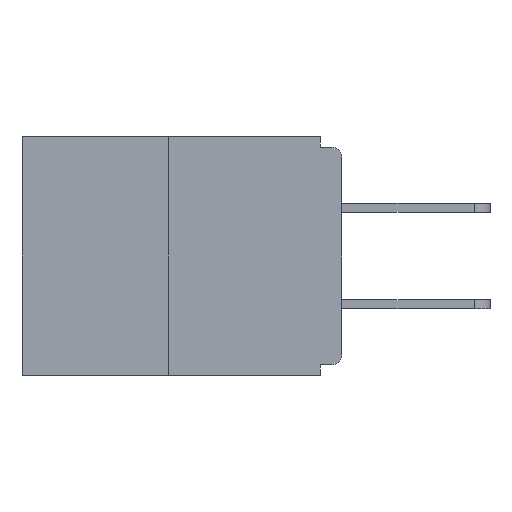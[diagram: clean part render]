
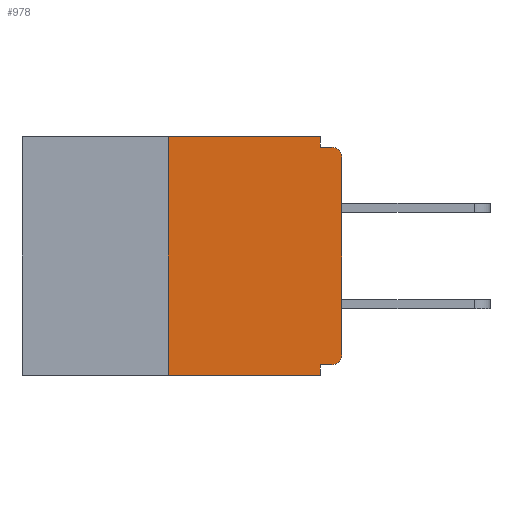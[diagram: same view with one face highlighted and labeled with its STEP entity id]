
A CAD part, left-side view. The second image highlights one B-rep face of the part: STEP entity #978.
In plain terms, the highlighted planar face has unit normal (-1, 0, 0).
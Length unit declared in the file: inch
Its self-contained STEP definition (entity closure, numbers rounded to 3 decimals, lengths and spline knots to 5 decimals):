
#153 = CARTESIAN_POINT ( 'NONE',  ( 0., 0.031, -0.343 ) ) ;
#158 = CARTESIAN_POINT ( 'NONE',  ( 0., 0.25, 0. ) ) ;
#217 = CIRCLE ( 'NONE', #15410, 0.015 ) ;
#261 = DIRECTION ( 'NONE',  ( -1., 0., 0. ) ) ;
#465 = EDGE_CURVE ( 'NONE', #6177, #3303, #217, .T. ) ;
#733 = CARTESIAN_POINT ( 'NONE',  ( 0., 0.46, 0. ) ) ;
#875 = LINE ( 'NONE', #19701, #16586 ) ;
#978 = ADVANCED_FACE ( 'NONE', ( #18193 ), #2371, .F. ) ;
#1172 = LINE ( 'NONE', #12263, #5443 ) ;
#1316 = DIRECTION ( 'NONE',  ( -1., 0., 0. ) ) ;
#1466 = DIRECTION ( 'NONE',  ( 0., -1., 0. ) ) ;
#2028 = VECTOR ( 'NONE', #12916, 39.37008 ) ;
#2207 = VERTEX_POINT ( 'NONE', #18296 ) ;
#2371 = PLANE ( 'NONE',  #22600 ) ;
#3303 = VERTEX_POINT ( 'NONE', #15608 ) ;
#3715 = VERTEX_POINT ( 'NONE', #8176 ) ;
#4021 = CARTESIAN_POINT ( 'NONE',  ( 0., 0.031, -0.015 ) ) ;
#4206 = DIRECTION ( 'NONE',  ( 0., 0., -1. ) ) ;
#4287 = DIRECTION ( 'NONE',  ( 0., 0., 1. ) ) ;
#4535 = EDGE_CURVE ( 'NONE', #2207, #3715, #1172, .T. ) ;
#4591 = LINE ( 'NONE', #19845, #22901 ) ;
#4742 = VECTOR ( 'NONE', #4287, 39.37008 ) ;
#4853 = VECTOR ( 'NONE', #22269, 39.37008 ) ;
#4872 = ORIENTED_EDGE ( 'NONE', *, *, #4535, .T. ) ;
#5381 = EDGE_CURVE ( 'NONE', #11959, #3715, #23169, .T. ) ;
#5443 = VECTOR ( 'NONE', #17762, 39.37008 ) ;
#5490 = ORIENTED_EDGE ( 'NONE', *, *, #19699, .F. ) ;
#5657 = VERTEX_POINT ( 'NONE', #13048 ) ;
#5680 = ORIENTED_EDGE ( 'NONE', *, *, #15612, .F. ) ;
#6177 = VERTEX_POINT ( 'NONE', #10627 ) ;
#6433 = CARTESIAN_POINT ( 'NONE',  ( 0., 0., -0.015 ) ) ;
#6871 = LINE ( 'NONE', #11267, #2028 ) ;
#7163 = CARTESIAN_POINT ( 'NONE',  ( 0., 0., -0.313 ) ) ;
#8176 = CARTESIAN_POINT ( 'NONE',  ( 0., 0.031, -0.343 ) ) ;
#8736 = DIRECTION ( 'NONE',  ( 0., 0., 1. ) ) ;
#8847 = CARTESIAN_POINT ( 'NONE',  ( 0., 0.031, -0.328 ) ) ;
#9105 = DIRECTION ( 'NONE',  ( 0., 1., 0. ) ) ;
#9174 = LINE ( 'NONE', #6433, #23471 ) ;
#9337 = LINE ( 'NONE', #21830, #23357 ) ;
#10178 = LINE ( 'NONE', #17390, #4742 ) ;
#10183 = DIRECTION ( 'NONE',  ( 0., -1., 0. ) ) ;
#10627 = CARTESIAN_POINT ( 'NONE',  ( 0., 0., -0.03 ) ) ;
#10668 = CARTESIAN_POINT ( 'NONE',  ( 0., 0.015, -0.313 ) ) ;
#11267 = CARTESIAN_POINT ( 'NONE',  ( 0., 0.031, 0. ) ) ;
#11917 = ORIENTED_EDGE ( 'NONE', *, *, #19468, .T. ) ;
#11959 = VERTEX_POINT ( 'NONE', #8847 ) ;
#12113 = DIRECTION ( 'NONE',  ( 0., 0., -1. ) ) ;
#12223 = CIRCLE ( 'NONE', #15354, 0.015 ) ;
#12263 = CARTESIAN_POINT ( 'NONE',  ( 0., 0.46, -0.343 ) ) ;
#12916 = DIRECTION ( 'NONE',  ( 0., 0., -1. ) ) ;
#12922 = ORIENTED_EDGE ( 'NONE', *, *, #16688, .F. ) ;
#13048 = CARTESIAN_POINT ( 'NONE',  ( 0., 0.031, 0. ) ) ;
#13144 = VERTEX_POINT ( 'NONE', #4021 ) ;
#14744 = EDGE_CURVE ( 'NONE', #5657, #13144, #6871, .T. ) ;
#15126 = EDGE_CURVE ( 'NONE', #16320, #6177, #875, .T. ) ;
#15354 = AXIS2_PLACEMENT_3D ( 'NONE', #10668, #1316, #12113 ) ;
#15410 = AXIS2_PLACEMENT_3D ( 'NONE', #18471, #261, #21910 ) ;
#15608 = CARTESIAN_POINT ( 'NONE',  ( 0., 0.015, -0.015 ) ) ;
#15612 = EDGE_CURVE ( 'NONE', #23091, #5657, #4591, .T. ) ;
#16320 = VERTEX_POINT ( 'NONE', #7163 ) ;
#16586 = VECTOR ( 'NONE', #8736, 39.37008 ) ;
#16688 = EDGE_CURVE ( 'NONE', #13144, #3303, #9174, .T. ) ;
#17390 = CARTESIAN_POINT ( 'NONE',  ( 0., 0.25, 0. ) ) ;
#17762 = DIRECTION ( 'NONE',  ( 0., -1., 0. ) ) ;
#18193 = FACE_OUTER_BOUND ( 'NONE', #23202, .T. ) ;
#18296 = CARTESIAN_POINT ( 'NONE',  ( 0., 0.25, -0.343 ) ) ;
#18396 = VERTEX_POINT ( 'NONE', #23648 ) ;
#18471 = CARTESIAN_POINT ( 'NONE',  ( 0., 0.015, -0.03 ) ) ;
#19468 = EDGE_CURVE ( 'NONE', #18396, #16320, #12223, .T. ) ;
#19576 = ORIENTED_EDGE ( 'NONE', *, *, #465, .T. ) ;
#19699 = EDGE_CURVE ( 'NONE', #18396, #11959, #9337, .T. ) ;
#19701 = CARTESIAN_POINT ( 'NONE',  ( 0., 0., 0. ) ) ;
#19845 = CARTESIAN_POINT ( 'NONE',  ( 0., 0.46, 0. ) ) ;
#20379 = ORIENTED_EDGE ( 'NONE', *, *, #14744, .F. ) ;
#20391 = ORIENTED_EDGE ( 'NONE', *, *, #5381, .F. ) ;
#20691 = DIRECTION ( 'NONE',  ( 1., 0., 0. ) ) ;
#20763 = EDGE_CURVE ( 'NONE', #2207, #23091, #10178, .T. ) ;
#20930 = ORIENTED_EDGE ( 'NONE', *, *, #15126, .T. ) ;
#21706 = ORIENTED_EDGE ( 'NONE', *, *, #20763, .F. ) ;
#21830 = CARTESIAN_POINT ( 'NONE',  ( 0., 0., -0.328 ) ) ;
#21910 = DIRECTION ( 'NONE',  ( 0., 0., -1. ) ) ;
#22269 = DIRECTION ( 'NONE',  ( 0., 0., -1. ) ) ;
#22600 = AXIS2_PLACEMENT_3D ( 'NONE', #733, #20691, #4206 ) ;
#22901 = VECTOR ( 'NONE', #1466, 39.37008 ) ;
#23091 = VERTEX_POINT ( 'NONE', #158 ) ;
#23169 = LINE ( 'NONE', #153, #4853 ) ;
#23202 = EDGE_LOOP ( 'NONE', ( #5680, #21706, #4872, #20391, #5490, #11917, #20930, #19576, #12922, #20379 ) ) ;
#23357 = VECTOR ( 'NONE', #9105, 39.37008 ) ;
#23471 = VECTOR ( 'NONE', #10183, 39.37008 ) ;
#23648 = CARTESIAN_POINT ( 'NONE',  ( 0., 0.015, -0.328 ) ) ;
